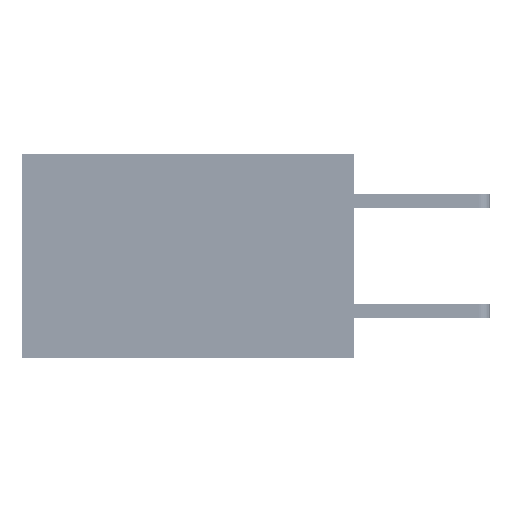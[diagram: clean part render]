
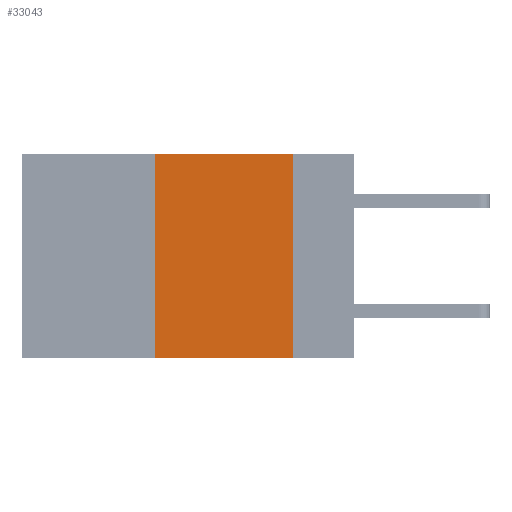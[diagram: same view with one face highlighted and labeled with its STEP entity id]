
A CAD part, left-side view. The second image highlights one B-rep face of the part: STEP entity #33043.
In plain terms, the highlighted planar face has unit normal (-1, 0, 0).
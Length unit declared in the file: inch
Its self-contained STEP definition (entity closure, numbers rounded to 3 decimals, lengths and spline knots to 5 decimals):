
#201 = DIRECTION ( 'NONE',  ( 0., -1., 0. ) ) ;
#1635 = EDGE_CURVE ( 'NONE', #20621, #38175, #35635, .T. ) ;
#2435 = DIRECTION ( 'NONE',  ( 0., 0., 1. ) ) ;
#4513 = EDGE_LOOP ( 'NONE', ( #35457, #8001, #29139, #13554 ) ) ;
#5223 = CARTESIAN_POINT ( 'NONE',  ( 0., 0.11, 0. ) ) ;
#8001 = ORIENTED_EDGE ( 'NONE', *, *, #41319, .F. ) ;
#11215 = DIRECTION ( 'NONE',  ( 0., -1., 0. ) ) ;
#12314 = VERTEX_POINT ( 'NONE', #18854 ) ;
#13554 = ORIENTED_EDGE ( 'NONE', *, *, #1635, .T. ) ;
#14617 = PLANE ( 'NONE',  #38802 ) ;
#16650 = VECTOR ( 'NONE', #11215, 39.37008 ) ;
#16751 = CARTESIAN_POINT ( 'NONE',  ( 0., 0.11, -0.37 ) ) ;
#17142 = CARTESIAN_POINT ( 'NONE',  ( 0., 0.6, 0. ) ) ;
#18552 = LINE ( 'NONE', #31509, #25277 ) ;
#18854 = CARTESIAN_POINT ( 'NONE',  ( 0., 0.36, 0. ) ) ;
#19623 = VECTOR ( 'NONE', #31739, 39.37008 ) ;
#20621 = VERTEX_POINT ( 'NONE', #32694 ) ;
#22182 = LINE ( 'NONE', #5223, #19623 ) ;
#25099 = VECTOR ( 'NONE', #201, 39.37008 ) ;
#25277 = VECTOR ( 'NONE', #2435, 39.37008 ) ;
#25359 = EDGE_CURVE ( 'NONE', #38521, #38175, #22182, .T. ) ;
#27565 = DIRECTION ( 'NONE',  ( 1., 0., 0. ) ) ;
#28404 = CARTESIAN_POINT ( 'NONE',  ( 0., 0.11, 0. ) ) ;
#29139 = ORIENTED_EDGE ( 'NONE', *, *, #34528, .F. ) ;
#31509 = CARTESIAN_POINT ( 'NONE',  ( 0., 0.36, 0. ) ) ;
#31739 = DIRECTION ( 'NONE',  ( 0., 0., -1. ) ) ;
#32694 = CARTESIAN_POINT ( 'NONE',  ( 0., 0.36, -0.37 ) ) ;
#33043 = ADVANCED_FACE ( 'NONE', ( #34352 ), #14617, .F. ) ;
#34352 = FACE_OUTER_BOUND ( 'NONE', #4513, .T. ) ;
#34528 = EDGE_CURVE ( 'NONE', #20621, #12314, #18552, .T. ) ;
#35457 = ORIENTED_EDGE ( 'NONE', *, *, #25359, .F. ) ;
#35635 = LINE ( 'NONE', #41809, #25099 ) ;
#38175 = VERTEX_POINT ( 'NONE', #16751 ) ;
#38521 = VERTEX_POINT ( 'NONE', #28404 ) ;
#38802 = AXIS2_PLACEMENT_3D ( 'NONE', #40944, #27565, #40524 ) ;
#39669 = LINE ( 'NONE', #17142, #16650 ) ;
#40524 = DIRECTION ( 'NONE',  ( 0., 0., -1. ) ) ;
#40944 = CARTESIAN_POINT ( 'NONE',  ( 0., 0.6, 0. ) ) ;
#41319 = EDGE_CURVE ( 'NONE', #12314, #38521, #39669, .T. ) ;
#41809 = CARTESIAN_POINT ( 'NONE',  ( 0., 0.6, -0.37 ) ) ;
